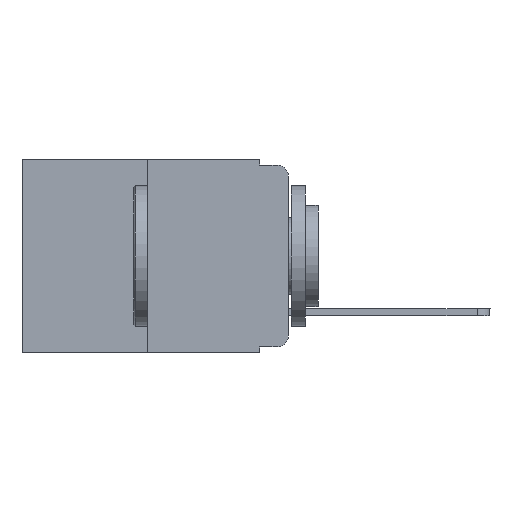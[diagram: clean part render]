
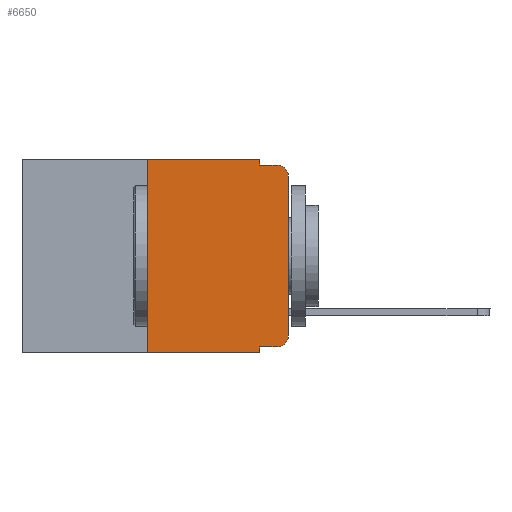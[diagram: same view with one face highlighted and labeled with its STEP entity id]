
A CAD part, left-side view. The second image highlights one B-rep face of the part: STEP entity #6650.
In plain terms, the highlighted planar face has unit normal (-1, 0, 0).
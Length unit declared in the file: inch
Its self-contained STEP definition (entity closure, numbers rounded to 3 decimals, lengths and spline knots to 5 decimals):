
#239 = DIRECTION ( 'NONE',  ( -1., 0., 0. ) ) ;
#269 = CARTESIAN_POINT ( 'NONE',  ( 0., 0.25, 0. ) ) ;
#297 = LINE ( 'NONE', #22371, #5307 ) ;
#486 = ORIENTED_EDGE ( 'NONE', *, *, #5573, .T. ) ;
#765 = CIRCLE ( 'NONE', #3647, 0.02 ) ;
#1032 = LINE ( 'NONE', #2839, #10532 ) ;
#1090 = CARTESIAN_POINT ( 'NONE',  ( 0., 0.051, -0.333 ) ) ;
#1178 = EDGE_CURVE ( 'NONE', #8572, #1905, #10847, .T. ) ;
#1252 = VERTEX_POINT ( 'NONE', #6189 ) ;
#1905 = VERTEX_POINT ( 'NONE', #7373 ) ;
#1974 = DIRECTION ( 'NONE',  ( 0., 0., -1. ) ) ;
#2613 = ORIENTED_EDGE ( 'NONE', *, *, #6803, .T. ) ;
#2635 = EDGE_CURVE ( 'NONE', #15868, #9981, #10711, .T. ) ;
#2708 = EDGE_CURVE ( 'NONE', #9635, #20588, #297, .T. ) ;
#2839 = CARTESIAN_POINT ( 'NONE',  ( 0., 0.25, 0. ) ) ;
#3013 = CARTESIAN_POINT ( 'NONE',  ( 0., 0.051, -0.01 ) ) ;
#3215 = AXIS2_PLACEMENT_3D ( 'NONE', #15747, #239, #20938 ) ;
#3647 = AXIS2_PLACEMENT_3D ( 'NONE', #6963, #8777, #13877 ) ;
#3795 = DIRECTION ( 'NONE',  ( 0., -1., 0. ) ) ;
#3804 = CARTESIAN_POINT ( 'NONE',  ( 0., 0.051, 0. ) ) ;
#5285 = CARTESIAN_POINT ( 'NONE',  ( 0., 0.051, -0.01 ) ) ;
#5293 = LINE ( 'NONE', #3804, #8449 ) ;
#5307 = VECTOR ( 'NONE', #15468, 39.37008 ) ;
#5573 = EDGE_CURVE ( 'NONE', #20588, #6706, #10078, .T. ) ;
#6189 = CARTESIAN_POINT ( 'NONE',  ( 0., 0.051, -0.343 ) ) ;
#6584 = EDGE_LOOP ( 'NONE', ( #2613, #21340, #16591, #13071, #7264, #17362, #14301, #7378, #19973, #486 ) ) ;
#6650 = ADVANCED_FACE ( 'NONE', ( #10237 ), #10465, .F. ) ;
#6706 = VERTEX_POINT ( 'NONE', #17994 ) ;
#6803 = EDGE_CURVE ( 'NONE', #6706, #9409, #11553, .T. ) ;
#6858 = EDGE_CURVE ( 'NONE', #17983, #8572, #1032, .T. ) ;
#6963 = CARTESIAN_POINT ( 'NONE',  ( 0., 0.02, -0.03 ) ) ;
#7264 = ORIENTED_EDGE ( 'NONE', *, *, #1178, .F. ) ;
#7319 = CARTESIAN_POINT ( 'NONE',  ( 0., 0.473, -0.343 ) ) ;
#7325 = LINE ( 'NONE', #17390, #12028 ) ;
#7373 = CARTESIAN_POINT ( 'NONE',  ( 0., 0.051, 0. ) ) ;
#7378 = ORIENTED_EDGE ( 'NONE', *, *, #9410, .F. ) ;
#7481 = CARTESIAN_POINT ( 'NONE',  ( 0., 0.02, -0.333 ) ) ;
#8158 = CARTESIAN_POINT ( 'NONE',  ( 0., 0., 0. ) ) ;
#8363 = EDGE_CURVE ( 'NONE', #17983, #1252, #17829, .T. ) ;
#8449 = VECTOR ( 'NONE', #18970, 39.37008 ) ;
#8572 = VERTEX_POINT ( 'NONE', #269 ) ;
#8597 = EDGE_CURVE ( 'NONE', #9409, #9981, #765, .T. ) ;
#8777 = DIRECTION ( 'NONE',  ( -1., 0., 0. ) ) ;
#9175 = VECTOR ( 'NONE', #18182, 39.37008 ) ;
#9383 = EDGE_CURVE ( 'NONE', #1905, #15868, #7325, .T. ) ;
#9409 = VERTEX_POINT ( 'NONE', #20676 ) ;
#9410 = EDGE_CURVE ( 'NONE', #9635, #1252, #5293, .T. ) ;
#9462 = DIRECTION ( 'NONE',  ( 0., -1., 0. ) ) ;
#9635 = VERTEX_POINT ( 'NONE', #1090 ) ;
#9950 = DIRECTION ( 'NONE',  ( 0., 0., -1. ) ) ;
#9981 = VERTEX_POINT ( 'NONE', #21317 ) ;
#10078 = CIRCLE ( 'NONE', #3215, 0.02 ) ;
#10237 = FACE_OUTER_BOUND ( 'NONE', #6584, .T. ) ;
#10465 = PLANE ( 'NONE',  #15953 ) ;
#10532 = VECTOR ( 'NONE', #14725, 39.37008 ) ;
#10711 = LINE ( 'NONE', #5285, #17557 ) ;
#10847 = LINE ( 'NONE', #16372, #9175 ) ;
#11217 = DIRECTION ( 'NONE',  ( 0., 0., 1. ) ) ;
#11553 = LINE ( 'NONE', #8158, #17395 ) ;
#12028 = VECTOR ( 'NONE', #9950, 39.37008 ) ;
#13071 = ORIENTED_EDGE ( 'NONE', *, *, #9383, .F. ) ;
#13877 = DIRECTION ( 'NONE',  ( 0., 0., -1. ) ) ;
#14301 = ORIENTED_EDGE ( 'NONE', *, *, #8363, .T. ) ;
#14466 = CARTESIAN_POINT ( 'NONE',  ( 0., 0.25, -0.343 ) ) ;
#14725 = DIRECTION ( 'NONE',  ( 0., 0., 1. ) ) ;
#15171 = VECTOR ( 'NONE', #9462, 39.37008 ) ;
#15468 = DIRECTION ( 'NONE',  ( 0., -1., 0. ) ) ;
#15747 = CARTESIAN_POINT ( 'NONE',  ( 0., 0.02, -0.313 ) ) ;
#15775 = DIRECTION ( 'NONE',  ( 1., 0., 0. ) ) ;
#15868 = VERTEX_POINT ( 'NONE', #3013 ) ;
#15953 = AXIS2_PLACEMENT_3D ( 'NONE', #17472, #15775, #1974 ) ;
#16372 = CARTESIAN_POINT ( 'NONE',  ( 0., 0.473, 0. ) ) ;
#16591 = ORIENTED_EDGE ( 'NONE', *, *, #2635, .F. ) ;
#17362 = ORIENTED_EDGE ( 'NONE', *, *, #6858, .F. ) ;
#17390 = CARTESIAN_POINT ( 'NONE',  ( 0., 0.051, 0. ) ) ;
#17395 = VECTOR ( 'NONE', #11217, 39.37008 ) ;
#17472 = CARTESIAN_POINT ( 'NONE',  ( 0., 0.473, 0. ) ) ;
#17557 = VECTOR ( 'NONE', #3795, 39.37008 ) ;
#17829 = LINE ( 'NONE', #7319, #15171 ) ;
#17983 = VERTEX_POINT ( 'NONE', #14466 ) ;
#17994 = CARTESIAN_POINT ( 'NONE',  ( 0., 0., -0.313 ) ) ;
#18182 = DIRECTION ( 'NONE',  ( 0., -1., 0. ) ) ;
#18970 = DIRECTION ( 'NONE',  ( 0., 0., -1. ) ) ;
#19973 = ORIENTED_EDGE ( 'NONE', *, *, #2708, .T. ) ;
#20588 = VERTEX_POINT ( 'NONE', #7481 ) ;
#20676 = CARTESIAN_POINT ( 'NONE',  ( 0., 0., -0.03 ) ) ;
#20938 = DIRECTION ( 'NONE',  ( 0., 0., -1. ) ) ;
#21317 = CARTESIAN_POINT ( 'NONE',  ( 0., 0.02, -0.01 ) ) ;
#21340 = ORIENTED_EDGE ( 'NONE', *, *, #8597, .T. ) ;
#22371 = CARTESIAN_POINT ( 'NONE',  ( 0., 0.051, -0.333 ) ) ;
